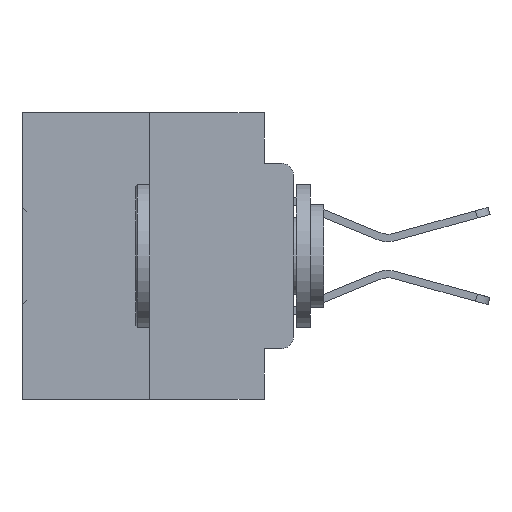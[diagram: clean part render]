
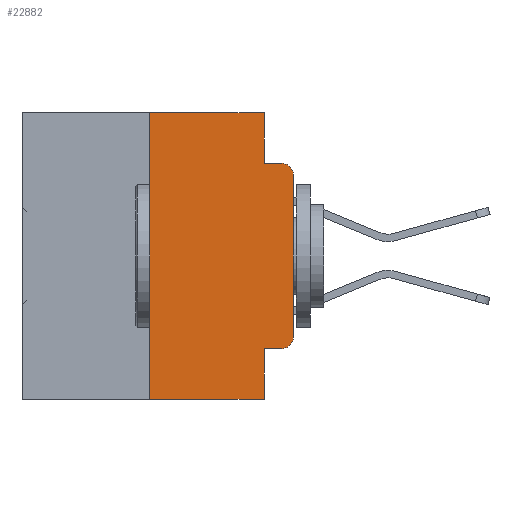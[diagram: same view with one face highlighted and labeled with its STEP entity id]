
A CAD part, left-side view. The second image highlights one B-rep face of the part: STEP entity #22882.
In plain terms, the highlighted planar face has unit normal (-1, 0, 0).
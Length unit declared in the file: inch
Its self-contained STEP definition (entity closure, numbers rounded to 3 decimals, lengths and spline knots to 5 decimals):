
#1081 = ORIENTED_EDGE ( 'NONE', *, *, #17654, .T. ) ;
#1170 = DIRECTION ( 'NONE',  ( 0., -1., 0. ) ) ;
#1262 = DIRECTION ( 'NONE',  ( 0., 0., -1. ) ) ;
#1934 = LINE ( 'NONE', #34312, #22616 ) ;
#2467 = ORIENTED_EDGE ( 'NONE', *, *, #15072, .F. ) ;
#2540 = VERTEX_POINT ( 'NONE', #21276 ) ;
#3288 = VECTOR ( 'NONE', #23039, 39.37008 ) ;
#3661 = EDGE_CURVE ( 'NONE', #10131, #4785, #21595, .T. ) ;
#3809 = VERTEX_POINT ( 'NONE', #29045 ) ;
#4064 = CARTESIAN_POINT ( 'NONE',  ( 0., 0.051, 0. ) ) ;
#4167 = LINE ( 'NONE', #17606, #3288 ) ;
#4218 = DIRECTION ( 'NONE',  ( 0., 0., 1. ) ) ;
#4354 = ORIENTED_EDGE ( 'NONE', *, *, #24342, .T. ) ;
#4785 = VERTEX_POINT ( 'NONE', #12753 ) ;
#4889 = VERTEX_POINT ( 'NONE', #14012 ) ;
#5388 = VECTOR ( 'NONE', #34968, 39.37008 ) ;
#5548 = EDGE_CURVE ( 'NONE', #4889, #15379, #11313, .T. ) ;
#5651 = VERTEX_POINT ( 'NONE', #26775 ) ;
#5688 = VECTOR ( 'NONE', #4218, 39.37008 ) ;
#5904 = VECTOR ( 'NONE', #13383, 39.37008 ) ;
#7288 = CARTESIAN_POINT ( 'NONE',  ( 0., 0., -0.1085 ) ) ;
#8041 = LINE ( 'NONE', #26053, #9826 ) ;
#8428 = ORIENTED_EDGE ( 'NONE', *, *, #34955, .T. ) ;
#9468 = DIRECTION ( 'NONE',  ( -1., 0., 0. ) ) ;
#9548 = VECTOR ( 'NONE', #1262, 39.37008 ) ;
#9712 = CARTESIAN_POINT ( 'NONE',  ( 0., 0.25, -0.5 ) ) ;
#9826 = VECTOR ( 'NONE', #23337, 39.37008 ) ;
#10079 = ORIENTED_EDGE ( 'NONE', *, *, #23211, .T. ) ;
#10131 = VERTEX_POINT ( 'NONE', #9712 ) ;
#10287 = ORIENTED_EDGE ( 'NONE', *, *, #3661, .F. ) ;
#10550 = CARTESIAN_POINT ( 'NONE',  ( 0., 0.051, -0.4115 ) ) ;
#11313 = LINE ( 'NONE', #4064, #9548 ) ;
#11915 = DIRECTION ( 'NONE',  ( 1., 0., 0. ) ) ;
#12381 = CARTESIAN_POINT ( 'NONE',  ( 0., 0.02, -0.3915 ) ) ;
#12753 = CARTESIAN_POINT ( 'NONE',  ( 0., 0.25, 0. ) ) ;
#13233 = CARTESIAN_POINT ( 'NONE',  ( 0., 0.02, -0.0885 ) ) ;
#13383 = DIRECTION ( 'NONE',  ( 0., -1., 0. ) ) ;
#13447 = LINE ( 'NONE', #10550, #5904 ) ;
#13936 = VECTOR ( 'NONE', #24036, 39.37008 ) ;
#14012 = CARTESIAN_POINT ( 'NONE',  ( 0., 0.051, 0. ) ) ;
#15072 = EDGE_CURVE ( 'NONE', #15379, #35142, #28614, .T. ) ;
#15258 = DIRECTION ( 'NONE',  ( 0., 0., -1. ) ) ;
#15379 = VERTEX_POINT ( 'NONE', #33431 ) ;
#16818 = EDGE_CURVE ( 'NONE', #4785, #4889, #8041, .T. ) ;
#16961 = EDGE_CURVE ( 'NONE', #20107, #35142, #25939, .T. ) ;
#17511 = PLANE ( 'NONE',  #33730 ) ;
#17606 = CARTESIAN_POINT ( 'NONE',  ( 0., 0.051, 0. ) ) ;
#17654 = EDGE_CURVE ( 'NONE', #25505, #5651, #19548, .T. ) ;
#19502 = ORIENTED_EDGE ( 'NONE', *, *, #16818, .F. ) ;
#19548 = CIRCLE ( 'NONE', #27508, 0.02 ) ;
#20107 = VERTEX_POINT ( 'NONE', #7288 ) ;
#20423 = LINE ( 'NONE', #26872, #5388 ) ;
#21276 = CARTESIAN_POINT ( 'NONE',  ( 0., 0.051, -0.4115 ) ) ;
#21595 = LINE ( 'NONE', #35231, #5688 ) ;
#22616 = VECTOR ( 'NONE', #1170, 39.37008 ) ;
#22882 = ADVANCED_FACE ( 'NONE', ( #33620 ), #17511, .F. ) ;
#23039 = DIRECTION ( 'NONE',  ( 0., 0., -1. ) ) ;
#23211 = EDGE_CURVE ( 'NONE', #2540, #25505, #13447, .T. ) ;
#23337 = DIRECTION ( 'NONE',  ( 0., -1., 0. ) ) ;
#23715 = EDGE_LOOP ( 'NONE', ( #4354, #34261, #2467, #32516, #19502, #10287, #8428, #28099, #10079, #1081 ) ) ;
#24036 = DIRECTION ( 'NONE',  ( 0., -1., 0. ) ) ;
#24155 = CARTESIAN_POINT ( 'NONE',  ( 0., 0.051, -0.0885 ) ) ;
#24342 = EDGE_CURVE ( 'NONE', #5651, #20107, #20423, .T. ) ;
#25242 = AXIS2_PLACEMENT_3D ( 'NONE', #26148, #9468, #28858 ) ;
#25505 = VERTEX_POINT ( 'NONE', #34417 ) ;
#25939 = CIRCLE ( 'NONE', #25242, 0.02 ) ;
#26053 = CARTESIAN_POINT ( 'NONE',  ( 0., 0.473, 0. ) ) ;
#26148 = CARTESIAN_POINT ( 'NONE',  ( 0., 0.02, -0.1085 ) ) ;
#26775 = CARTESIAN_POINT ( 'NONE',  ( 0., 0., -0.3915 ) ) ;
#26872 = CARTESIAN_POINT ( 'NONE',  ( 0., 0., 0. ) ) ;
#27508 = AXIS2_PLACEMENT_3D ( 'NONE', #12381, #31623, #15258 ) ;
#28099 = ORIENTED_EDGE ( 'NONE', *, *, #28652, .F. ) ;
#28377 = CARTESIAN_POINT ( 'NONE',  ( 0., 0.473, 0. ) ) ;
#28614 = LINE ( 'NONE', #24155, #13936 ) ;
#28652 = EDGE_CURVE ( 'NONE', #2540, #3809, #4167, .T. ) ;
#28858 = DIRECTION ( 'NONE',  ( 0., 0., -1. ) ) ;
#29045 = CARTESIAN_POINT ( 'NONE',  ( 0., 0.051, -0.5 ) ) ;
#31179 = DIRECTION ( 'NONE',  ( 0., 0., -1. ) ) ;
#31623 = DIRECTION ( 'NONE',  ( -1., 0., 0. ) ) ;
#32516 = ORIENTED_EDGE ( 'NONE', *, *, #5548, .F. ) ;
#33431 = CARTESIAN_POINT ( 'NONE',  ( 0., 0.051, -0.0885 ) ) ;
#33620 = FACE_OUTER_BOUND ( 'NONE', #23715, .T. ) ;
#33730 = AXIS2_PLACEMENT_3D ( 'NONE', #28377, #11915, #31179 ) ;
#34261 = ORIENTED_EDGE ( 'NONE', *, *, #16961, .T. ) ;
#34312 = CARTESIAN_POINT ( 'NONE',  ( 0., 0.473, -0.5 ) ) ;
#34417 = CARTESIAN_POINT ( 'NONE',  ( 0., 0.02, -0.4115 ) ) ;
#34955 = EDGE_CURVE ( 'NONE', #10131, #3809, #1934, .T. ) ;
#34968 = DIRECTION ( 'NONE',  ( 0., 0., 1. ) ) ;
#35142 = VERTEX_POINT ( 'NONE', #13233 ) ;
#35231 = CARTESIAN_POINT ( 'NONE',  ( 0., 0.25, 0. ) ) ;
